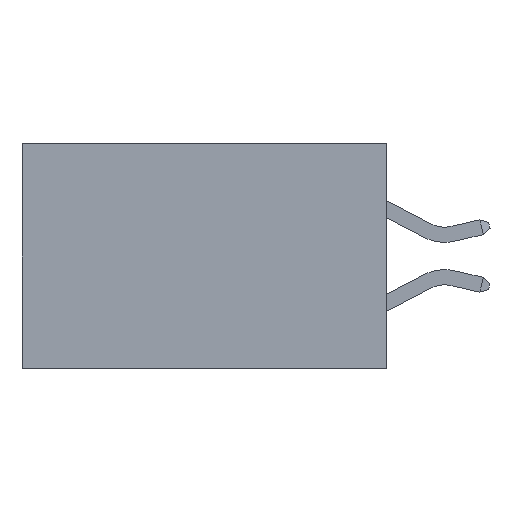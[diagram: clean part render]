
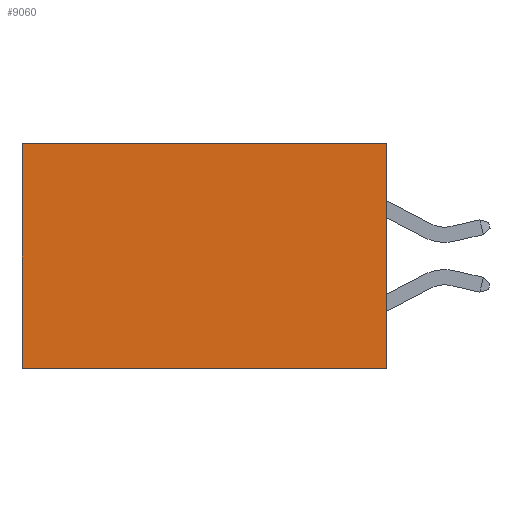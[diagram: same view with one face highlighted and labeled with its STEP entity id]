
A CAD part, left-side view. The second image highlights one B-rep face of the part: STEP entity #9060.
In plain terms, the highlighted planar face has unit normal (-1, 0, 0).
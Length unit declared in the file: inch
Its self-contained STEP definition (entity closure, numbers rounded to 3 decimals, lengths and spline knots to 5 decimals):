
#431 = ORIENTED_EDGE ( 'NONE', *, *, #537, .F. ) ;
#468 = DIRECTION ( 'NONE',  ( 0., 0., -1. ) ) ;
#537 = EDGE_CURVE ( 'NONE', #8894, #4140, #3572, .T. ) ;
#814 = VECTOR ( 'NONE', #4344, 39.37008 ) ;
#816 = CARTESIAN_POINT ( 'NONE',  ( 0.2615, 0.6, -0.37 ) ) ;
#894 = ORIENTED_EDGE ( 'NONE', *, *, #4048, .T. ) ;
#996 = ORIENTED_EDGE ( 'NONE', *, *, #5869, .F. ) ;
#1087 = CARTESIAN_POINT ( 'NONE',  ( 0.2615, 0., 0. ) ) ;
#1755 = ORIENTED_EDGE ( 'NONE', *, *, #6960, .T. ) ;
#1957 = CARTESIAN_POINT ( 'NONE',  ( 0.2615, 0., -0.37 ) ) ;
#2086 = LINE ( 'NONE', #2134, #8162 ) ;
#2128 = AXIS2_PLACEMENT_3D ( 'NONE', #1957, #7399, #468 ) ;
#2134 = CARTESIAN_POINT ( 'NONE',  ( 0.2615, 0., 0. ) ) ;
#2452 = CARTESIAN_POINT ( 'NONE',  ( 0.2615, 0.6, 0. ) ) ;
#2529 = VERTEX_POINT ( 'NONE', #2452 ) ;
#2746 = DIRECTION ( 'NONE',  ( 0., 0., -1. ) ) ;
#3337 = FACE_OUTER_BOUND ( 'NONE', #7753, .T. ) ;
#3572 = LINE ( 'NONE', #5871, #814 ) ;
#3607 = CARTESIAN_POINT ( 'NONE',  ( 0.2615, 0., -0.37 ) ) ;
#4048 = EDGE_CURVE ( 'NONE', #2529, #4140, #7606, .T. ) ;
#4140 = VERTEX_POINT ( 'NONE', #816 ) ;
#4344 = DIRECTION ( 'NONE',  ( 0., 1., 0. ) ) ;
#4869 = PLANE ( 'NONE',  #2128 ) ;
#5869 = EDGE_CURVE ( 'NONE', #6868, #8894, #8240, .T. ) ;
#5871 = CARTESIAN_POINT ( 'NONE',  ( 0.2615, 0., -0.37 ) ) ;
#6868 = VERTEX_POINT ( 'NONE', #1087 ) ;
#6899 = DIRECTION ( 'NONE',  ( 0., 1., 0. ) ) ;
#6944 = CARTESIAN_POINT ( 'NONE',  ( 0.2615, 0., -0.37 ) ) ;
#6960 = EDGE_CURVE ( 'NONE', #6868, #2529, #2086, .T. ) ;
#7399 = DIRECTION ( 'NONE',  ( 1., 0., 0. ) ) ;
#7606 = LINE ( 'NONE', #9135, #7781 ) ;
#7753 = EDGE_LOOP ( 'NONE', ( #894, #431, #996, #1755 ) ) ;
#7781 = VECTOR ( 'NONE', #8151, 39.37008 ) ;
#8151 = DIRECTION ( 'NONE',  ( 0., 0., -1. ) ) ;
#8162 = VECTOR ( 'NONE', #6899, 39.37008 ) ;
#8240 = LINE ( 'NONE', #3607, #8722 ) ;
#8722 = VECTOR ( 'NONE', #2746, 39.37008 ) ;
#8894 = VERTEX_POINT ( 'NONE', #6944 ) ;
#9060 = ADVANCED_FACE ( 'NONE', ( #3337 ), #4869, .F. ) ;
#9135 = CARTESIAN_POINT ( 'NONE',  ( 0.2615, 0.6, -0.37 ) ) ;
